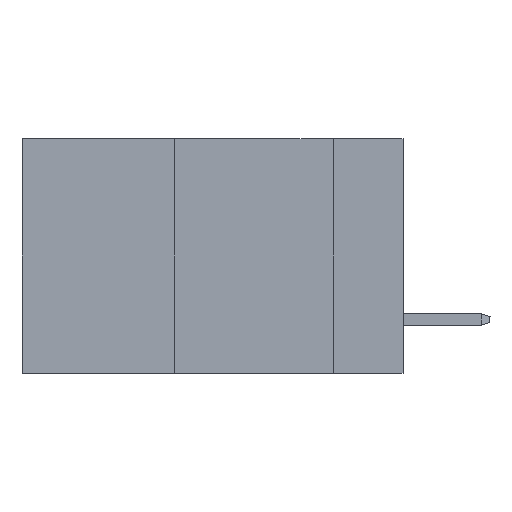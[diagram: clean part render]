
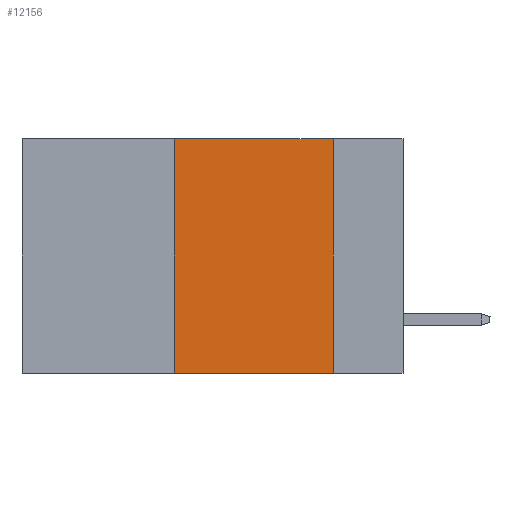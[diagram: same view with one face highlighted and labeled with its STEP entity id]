
A CAD part, left-side view. The second image highlights one B-rep face of the part: STEP entity #12156.
In plain terms, the highlighted planar face has unit normal (-1, 0, 0).
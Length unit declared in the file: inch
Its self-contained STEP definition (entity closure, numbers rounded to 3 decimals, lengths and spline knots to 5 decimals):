
#2294 = VERTEX_POINT ( 'NONE', #35231 ) ;
#3456 = LINE ( 'NONE', #27032, #27469 ) ;
#6837 = CARTESIAN_POINT ( 'NONE',  ( 0., 0.36, -0.37 ) ) ;
#7624 = VERTEX_POINT ( 'NONE', #35540 ) ;
#8504 = CARTESIAN_POINT ( 'NONE',  ( 0., 0.6, -0.37 ) ) ;
#12059 = DIRECTION ( 'NONE',  ( 0., -1., 0. ) ) ;
#12156 = ADVANCED_FACE ( 'NONE', ( #39545 ), #23981, .F. ) ;
#15604 = DIRECTION ( 'NONE',  ( 0., -1., 0. ) ) ;
#16098 = DIRECTION ( 'NONE',  ( 1., 0., 0. ) ) ;
#16361 = CARTESIAN_POINT ( 'NONE',  ( 0., 0.11, 0. ) ) ;
#16589 = CARTESIAN_POINT ( 'NONE',  ( 0., 0.36, 0. ) ) ;
#21339 = ORIENTED_EDGE ( 'NONE', *, *, #31275, .T. ) ;
#22302 = ORIENTED_EDGE ( 'NONE', *, *, #27797, .F. ) ;
#22730 = ORIENTED_EDGE ( 'NONE', *, *, #33756, .F. ) ;
#23469 = CARTESIAN_POINT ( 'NONE',  ( 0., 0.6, 0. ) ) ;
#23981 = PLANE ( 'NONE',  #34678 ) ;
#24234 = DIRECTION ( 'NONE',  ( 0., 0., -1. ) ) ;
#24299 = VERTEX_POINT ( 'NONE', #16589 ) ;
#27032 = CARTESIAN_POINT ( 'NONE',  ( 0., 0.6, 0. ) ) ;
#27365 = LINE ( 'NONE', #39379, #30354 ) ;
#27404 = VECTOR ( 'NONE', #24234, 39.37008 ) ;
#27469 = VECTOR ( 'NONE', #15604, 39.37008 ) ;
#27524 = LINE ( 'NONE', #16361, #27404 ) ;
#27797 = EDGE_CURVE ( 'NONE', #37693, #24299, #27365, .T. ) ;
#30354 = VECTOR ( 'NONE', #46762, 39.37008 ) ;
#30896 = LINE ( 'NONE', #8504, #46125 ) ;
#31275 = EDGE_CURVE ( 'NONE', #37693, #2294, #30896, .T. ) ;
#33452 = ORIENTED_EDGE ( 'NONE', *, *, #43604, .F. ) ;
#33756 = EDGE_CURVE ( 'NONE', #7624, #2294, #27524, .T. ) ;
#34678 = AXIS2_PLACEMENT_3D ( 'NONE', #23469, #16098, #42595 ) ;
#35231 = CARTESIAN_POINT ( 'NONE',  ( 0., 0.11, -0.37 ) ) ;
#35540 = CARTESIAN_POINT ( 'NONE',  ( 0., 0.11, 0. ) ) ;
#37693 = VERTEX_POINT ( 'NONE', #6837 ) ;
#39379 = CARTESIAN_POINT ( 'NONE',  ( 0., 0.36, 0. ) ) ;
#39545 = FACE_OUTER_BOUND ( 'NONE', #41451, .T. ) ;
#41451 = EDGE_LOOP ( 'NONE', ( #22730, #33452, #22302, #21339 ) ) ;
#42595 = DIRECTION ( 'NONE',  ( 0., 0., -1. ) ) ;
#43604 = EDGE_CURVE ( 'NONE', #24299, #7624, #3456, .T. ) ;
#46125 = VECTOR ( 'NONE', #12059, 39.37008 ) ;
#46762 = DIRECTION ( 'NONE',  ( 0., 0., 1. ) ) ;
